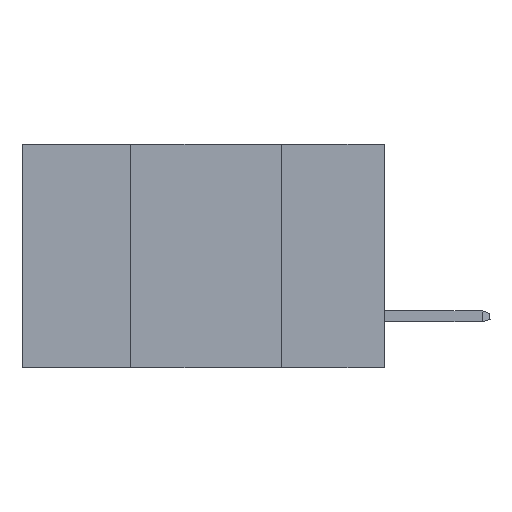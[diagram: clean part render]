
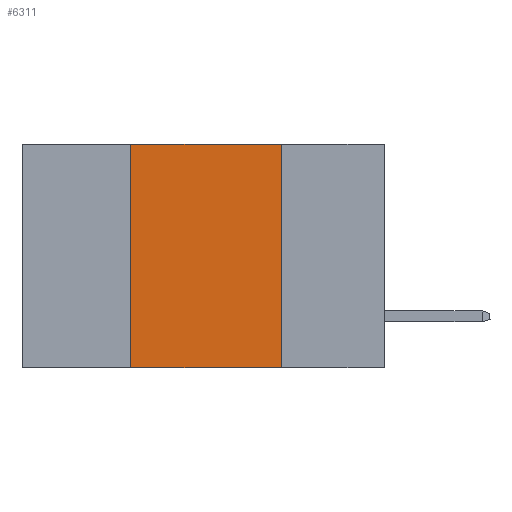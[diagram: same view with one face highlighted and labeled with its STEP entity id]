
A CAD part, left-side view. The second image highlights one B-rep face of the part: STEP entity #6311.
In plain terms, the highlighted planar face has unit normal (-1, 0, 0).
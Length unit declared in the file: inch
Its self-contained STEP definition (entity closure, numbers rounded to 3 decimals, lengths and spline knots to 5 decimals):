
#202 = VERTEX_POINT ( 'NONE', #10241 ) ;
#521 = EDGE_CURVE ( 'NONE', #202, #18173, #2407, .T. ) ;
#1761 = LINE ( 'NONE', #4115, #6923 ) ;
#2407 = LINE ( 'NONE', #30498, #28791 ) ;
#2746 = ORIENTED_EDGE ( 'NONE', *, *, #25836, .F. ) ;
#3001 = LINE ( 'NONE', #25798, #15240 ) ;
#3199 = EDGE_CURVE ( 'NONE', #18173, #22402, #3001, .T. ) ;
#3900 = CARTESIAN_POINT ( 'NONE',  ( 0., 0.6, -0.37 ) ) ;
#4115 = CARTESIAN_POINT ( 'NONE',  ( 0., 0.17, 0. ) ) ;
#5402 = EDGE_LOOP ( 'NONE', ( #2746, #14403, #20638, #12774 ) ) ;
#5820 = DIRECTION ( 'NONE',  ( 0., -1., 0. ) ) ;
#5827 = VECTOR ( 'NONE', #19076, 39.37008 ) ;
#6311 = ADVANCED_FACE ( 'NONE', ( #23978 ), #19204, .F. ) ;
#6923 = VECTOR ( 'NONE', #18959, 39.37008 ) ;
#9877 = CARTESIAN_POINT ( 'NONE',  ( 0., 0.42, 0. ) ) ;
#10241 = CARTESIAN_POINT ( 'NONE',  ( 0., 0.42, -0.37 ) ) ;
#10592 = CARTESIAN_POINT ( 'NONE',  ( 0., 0.17, 0. ) ) ;
#12774 = ORIENTED_EDGE ( 'NONE', *, *, #24621, .T. ) ;
#14096 = AXIS2_PLACEMENT_3D ( 'NONE', #31628, #29421, #16887 ) ;
#14403 = ORIENTED_EDGE ( 'NONE', *, *, #3199, .F. ) ;
#15240 = VECTOR ( 'NONE', #5820, 39.37008 ) ;
#16285 = VERTEX_POINT ( 'NONE', #16744 ) ;
#16744 = CARTESIAN_POINT ( 'NONE',  ( 0., 0.17, -0.37 ) ) ;
#16887 = DIRECTION ( 'NONE',  ( 0., 0., -1. ) ) ;
#18173 = VERTEX_POINT ( 'NONE', #9877 ) ;
#18959 = DIRECTION ( 'NONE',  ( 0., 0., -1. ) ) ;
#19076 = DIRECTION ( 'NONE',  ( 0., -1., 0. ) ) ;
#19204 = PLANE ( 'NONE',  #14096 ) ;
#20638 = ORIENTED_EDGE ( 'NONE', *, *, #521, .F. ) ;
#20761 = LINE ( 'NONE', #3900, #5827 ) ;
#22402 = VERTEX_POINT ( 'NONE', #10592 ) ;
#23102 = DIRECTION ( 'NONE',  ( 0., 0., 1. ) ) ;
#23978 = FACE_OUTER_BOUND ( 'NONE', #5402, .T. ) ;
#24621 = EDGE_CURVE ( 'NONE', #202, #16285, #20761, .T. ) ;
#25798 = CARTESIAN_POINT ( 'NONE',  ( 0., 0.6, 0. ) ) ;
#25836 = EDGE_CURVE ( 'NONE', #22402, #16285, #1761, .T. ) ;
#28791 = VECTOR ( 'NONE', #23102, 39.37008 ) ;
#29421 = DIRECTION ( 'NONE',  ( 1., 0., 0. ) ) ;
#30498 = CARTESIAN_POINT ( 'NONE',  ( 0., 0.42, 0. ) ) ;
#31628 = CARTESIAN_POINT ( 'NONE',  ( 0., 0.6, 0. ) ) ;
